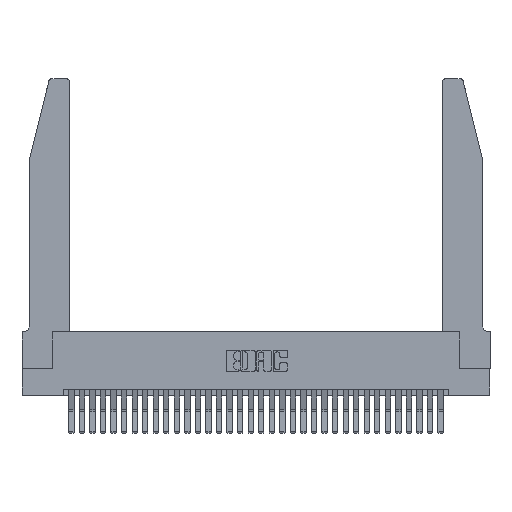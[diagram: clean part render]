
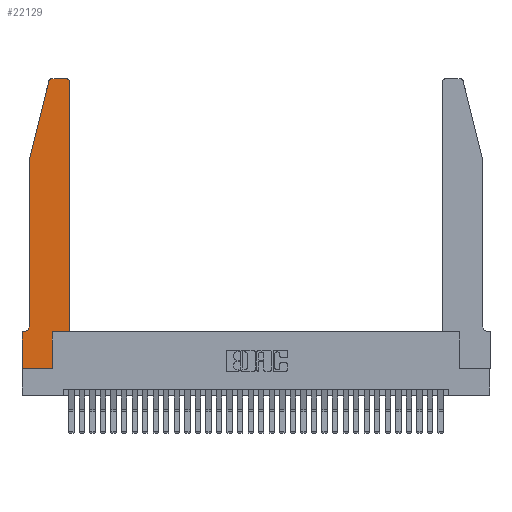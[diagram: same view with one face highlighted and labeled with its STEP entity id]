
A CAD part, top view. The second image highlights one B-rep face of the part: STEP entity #22129.
In plain terms, the highlighted planar face has unit normal (0, 0, 1).
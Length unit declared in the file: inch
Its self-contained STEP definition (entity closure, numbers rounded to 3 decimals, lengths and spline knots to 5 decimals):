
#96 = VECTOR ( 'NONE', #23324, 39.37008 ) ;
#466 = EDGE_CURVE ( 'NONE', #11093, #2232, #18171, .T. ) ;
#748 = ORIENTED_EDGE ( 'NONE', *, *, #12134, .T. ) ;
#962 = EDGE_CURVE ( 'NONE', #2232, #32111, #19140, .T. ) ;
#1030 = LINE ( 'NONE', #2956, #14317 ) ;
#1469 = DIRECTION ( 'NONE',  ( 1., 0., 0. ) ) ;
#2232 = VERTEX_POINT ( 'NONE', #16493 ) ;
#2562 = EDGE_CURVE ( 'NONE', #4805, #31727, #11262, .T. ) ;
#2918 = VECTOR ( 'NONE', #25388, 39.37008 ) ;
#2956 = CARTESIAN_POINT ( 'NONE',  ( 0.2605, 2.75, 0.37 ) ) ;
#3076 = VERTEX_POINT ( 'NONE', #22631 ) ;
#3270 = VECTOR ( 'NONE', #27650, 39.37008 ) ;
#3973 = EDGE_CURVE ( 'NONE', #12577, #25967, #33544, .T. ) ;
#4059 = ORIENTED_EDGE ( 'NONE', *, *, #962, .T. ) ;
#4293 = EDGE_CURVE ( 'NONE', #25967, #12340, #9867, .T. ) ;
#4338 = CARTESIAN_POINT ( 'NONE',  ( 0.4505, 0.35, 0.37 ) ) ;
#4627 = CARTESIAN_POINT ( 'NONE',  ( 0.25487, 2.72718, 0.37 ) ) ;
#4805 = VERTEX_POINT ( 'NONE', #28416 ) ;
#4869 = VERTEX_POINT ( 'NONE', #31155 ) ;
#5600 = DIRECTION ( 'NONE',  ( -1., 0., 0. ) ) ;
#7352 = VECTOR ( 'NONE', #7748, 39.37008 ) ;
#7748 = DIRECTION ( 'NONE',  ( 1., 0., 0. ) ) ;
#7819 = VERTEX_POINT ( 'NONE', #4627 ) ;
#8569 = CARTESIAN_POINT ( 'NONE',  ( 0.0055, 0.35, 0.37 ) ) ;
#9260 = DIRECTION ( 'NONE',  ( 0., -1., 0. ) ) ;
#9863 = ORIENTED_EDGE ( 'NONE', *, *, #26642, .T. ) ;
#9867 = CIRCLE ( 'NONE', #9999, 0.07 ) ;
#9999 = AXIS2_PLACEMENT_3D ( 'NONE', #26161, #10529, #28803 ) ;
#10529 = DIRECTION ( 'NONE',  ( 0., 0., -1. ) ) ;
#10654 = CARTESIAN_POINT ( 'NONE',  ( 0.4205, 2.75, 0.37 ) ) ;
#10717 = ORIENTED_EDGE ( 'NONE', *, *, #21789, .T. ) ;
#11093 = VERTEX_POINT ( 'NONE', #23086 ) ;
#11262 = LINE ( 'NONE', #15481, #31250 ) ;
#12063 = PLANE ( 'NONE',  #32858 ) ;
#12134 = EDGE_CURVE ( 'NONE', #31727, #14876, #13611, .T. ) ;
#12340 = VERTEX_POINT ( 'NONE', #8569 ) ;
#12380 = ORIENTED_EDGE ( 'NONE', *, *, #4293, .T. ) ;
#12577 = VERTEX_POINT ( 'NONE', #28479 ) ;
#13342 = CARTESIAN_POINT ( 'NONE',  ( 0.284, 2.72, 0.37 ) ) ;
#13350 = FACE_OUTER_BOUND ( 'NONE', #14813, .T. ) ;
#13611 = LINE ( 'NONE', #20814, #7352 ) ;
#14214 = LINE ( 'NONE', #20753, #96 ) ;
#14317 = VECTOR ( 'NONE', #5600, 39.37008 ) ;
#14813 = EDGE_LOOP ( 'NONE', ( #9863, #10717, #24610, #31536, #12380, #26225, #27866, #748, #15655, #29526, #31146, #4059 ) ) ;
#14876 = VERTEX_POINT ( 'NONE', #24838 ) ;
#15033 = DIRECTION ( 'NONE',  ( 1., 0., 0. ) ) ;
#15481 = CARTESIAN_POINT ( 'NONE',  ( 0., 0., 0.37 ) ) ;
#15655 = ORIENTED_EDGE ( 'NONE', *, *, #17689, .T. ) ;
#15943 = CARTESIAN_POINT ( 'NONE',  ( 0., 0., 0.37 ) ) ;
#15964 = DIRECTION ( 'NONE',  ( 1., 0., 0. ) ) ;
#16132 = CARTESIAN_POINT ( 'NONE',  ( 0.0755, 0.42, 0.37 ) ) ;
#16493 = CARTESIAN_POINT ( 'NONE',  ( 0.4505, 2.72, 0.37 ) ) ;
#16852 = EDGE_CURVE ( 'NONE', #4869, #11093, #27323, .T. ) ;
#17071 = CIRCLE ( 'NONE', #28281, 0.03 ) ;
#17330 = DIRECTION ( 'NONE',  ( 0., 0., 1. ) ) ;
#17689 = EDGE_CURVE ( 'NONE', #14876, #4869, #14214, .T. ) ;
#18171 = LINE ( 'NONE', #25401, #3270 ) ;
#18339 = AXIS2_PLACEMENT_3D ( 'NONE', #25259, #23028, #22899 ) ;
#18679 = LINE ( 'NONE', #22883, #2918 ) ;
#18834 = CARTESIAN_POINT ( 'NONE',  ( 0.0755, 0.35, 0.37 ) ) ;
#18982 = VECTOR ( 'NONE', #9260, 39.37008 ) ;
#19140 = CIRCLE ( 'NONE', #18339, 0.03 ) ;
#19491 = EDGE_CURVE ( 'NONE', #7819, #12577, #18679, .T. ) ;
#19631 = VECTOR ( 'NONE', #15033, 39.37008 ) ;
#20753 = CARTESIAN_POINT ( 'NONE',  ( 0.2865, 0.35, 0.37 ) ) ;
#20814 = CARTESIAN_POINT ( 'NONE',  ( 0., 0., 0.37 ) ) ;
#21454 = DIRECTION ( 'NONE',  ( -1., 0., 0. ) ) ;
#21789 = EDGE_CURVE ( 'NONE', #3076, #7819, #17071, .T. ) ;
#22129 = ADVANCED_FACE ( 'NONE', ( #13350 ), #12063, .T. ) ;
#22631 = CARTESIAN_POINT ( 'NONE',  ( 0.284, 2.75, 0.37 ) ) ;
#22883 = CARTESIAN_POINT ( 'NONE',  ( 0.0755, 2., 0.37 ) ) ;
#22899 = DIRECTION ( 'NONE',  ( 1., 0., 0. ) ) ;
#23028 = DIRECTION ( 'NONE',  ( 0., 0., 1. ) ) ;
#23086 = CARTESIAN_POINT ( 'NONE',  ( 0.4505, 0.35, 0.37 ) ) ;
#23324 = DIRECTION ( 'NONE',  ( 0., 1., 0. ) ) ;
#24610 = ORIENTED_EDGE ( 'NONE', *, *, #19491, .T. ) ;
#24838 = CARTESIAN_POINT ( 'NONE',  ( 0.2865, 0., 0.37 ) ) ;
#25259 = CARTESIAN_POINT ( 'NONE',  ( 0.4205, 2.72, 0.37 ) ) ;
#25388 = DIRECTION ( 'NONE',  ( -0.239, -0.971, 0. ) ) ;
#25401 = CARTESIAN_POINT ( 'NONE',  ( 0.4505, 0.35, 0.37 ) ) ;
#25967 = VERTEX_POINT ( 'NONE', #16132 ) ;
#26161 = CARTESIAN_POINT ( 'NONE',  ( 0.0055, 0.42, 0.37 ) ) ;
#26225 = ORIENTED_EDGE ( 'NONE', *, *, #31823, .T. ) ;
#26603 = VECTOR ( 'NONE', #21454, 39.37008 ) ;
#26642 = EDGE_CURVE ( 'NONE', #32111, #3076, #1030, .T. ) ;
#27323 = LINE ( 'NONE', #4338, #19631 ) ;
#27572 = CARTESIAN_POINT ( 'NONE',  ( 0.0755, 2., 0.37 ) ) ;
#27650 = DIRECTION ( 'NONE',  ( 0., 1., 0. ) ) ;
#27866 = ORIENTED_EDGE ( 'NONE', *, *, #2562, .T. ) ;
#28281 = AXIS2_PLACEMENT_3D ( 'NONE', #13342, #31560, #15964 ) ;
#28416 = CARTESIAN_POINT ( 'NONE',  ( 0., 0.35, 0.37 ) ) ;
#28454 = DIRECTION ( 'NONE',  ( 0., -1., 0. ) ) ;
#28479 = CARTESIAN_POINT ( 'NONE',  ( 0.0755, 2., 0.37 ) ) ;
#28803 = DIRECTION ( 'NONE',  ( -1., 0., 0. ) ) ;
#29526 = ORIENTED_EDGE ( 'NONE', *, *, #16852, .T. ) ;
#31146 = ORIENTED_EDGE ( 'NONE', *, *, #466, .T. ) ;
#31155 = CARTESIAN_POINT ( 'NONE',  ( 0.2865, 0.35, 0.37 ) ) ;
#31250 = VECTOR ( 'NONE', #28454, 39.37008 ) ;
#31536 = ORIENTED_EDGE ( 'NONE', *, *, #3973, .T. ) ;
#31560 = DIRECTION ( 'NONE',  ( 0., 0., 1. ) ) ;
#31727 = VERTEX_POINT ( 'NONE', #15943 ) ;
#31823 = EDGE_CURVE ( 'NONE', #12340, #4805, #33491, .T. ) ;
#32111 = VERTEX_POINT ( 'NONE', #10654 ) ;
#32858 = AXIS2_PLACEMENT_3D ( 'NONE', #32882, #17330, #1469 ) ;
#32882 = CARTESIAN_POINT ( 'NONE',  ( 0., 0.35, 0.37 ) ) ;
#33491 = LINE ( 'NONE', #18834, #26603 ) ;
#33544 = LINE ( 'NONE', #27572, #18982 ) ;
